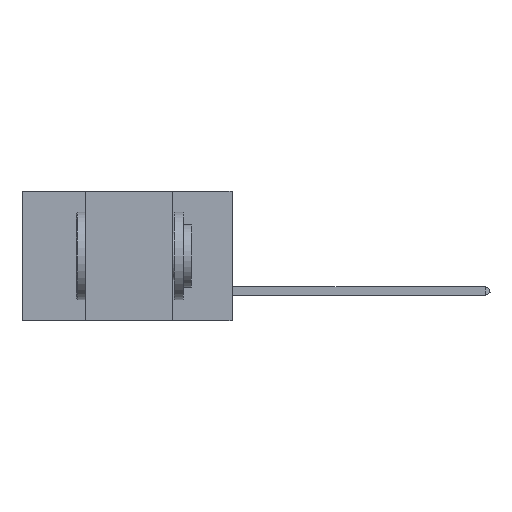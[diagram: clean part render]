
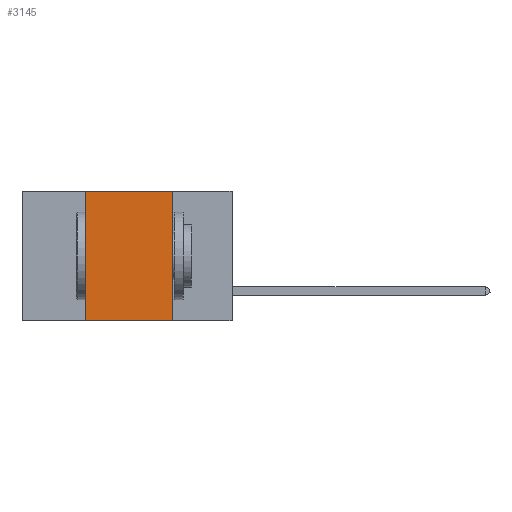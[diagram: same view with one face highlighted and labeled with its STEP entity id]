
A CAD part, left-side view. The second image highlights one B-rep face of the part: STEP entity #3145.
In plain terms, the highlighted planar face has unit normal (-1, 0, 0).
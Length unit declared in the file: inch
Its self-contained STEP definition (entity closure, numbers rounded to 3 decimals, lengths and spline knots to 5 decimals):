
#512 = DIRECTION ( 'NONE',  ( 0., -1., 0. ) ) ;
#902 = LINE ( 'NONE', #2764, #2570 ) ;
#1570 = FACE_OUTER_BOUND ( 'NONE', #9577, .T. ) ;
#2570 = VECTOR ( 'NONE', #2907, 39.37008 ) ;
#2736 = CARTESIAN_POINT ( 'NONE',  ( 0., 0.6, 0. ) ) ;
#2764 = CARTESIAN_POINT ( 'NONE',  ( 0., 0.42, 0. ) ) ;
#2907 = DIRECTION ( 'NONE',  ( 0., 0., 1. ) ) ;
#3134 = ORIENTED_EDGE ( 'NONE', *, *, #12017, .T. ) ;
#3145 = ADVANCED_FACE ( 'NONE', ( #1570 ), #3684, .F. ) ;
#3314 = LINE ( 'NONE', #2736, #4780 ) ;
#3684 = PLANE ( 'NONE',  #11522 ) ;
#4619 = ORIENTED_EDGE ( 'NONE', *, *, #10856, .F. ) ;
#4644 = CARTESIAN_POINT ( 'NONE',  ( 0., 0.17, -0.37 ) ) ;
#4731 = CARTESIAN_POINT ( 'NONE',  ( 0., 0.6, -0.37 ) ) ;
#4780 = VECTOR ( 'NONE', #10152, 39.37008 ) ;
#5534 = VERTEX_POINT ( 'NONE', #4644 ) ;
#5561 = EDGE_CURVE ( 'NONE', #11864, #7594, #3314, .T. ) ;
#6052 = LINE ( 'NONE', #4731, #12442 ) ;
#6476 = DIRECTION ( 'NONE',  ( 0., 0., -1. ) ) ;
#7594 = VERTEX_POINT ( 'NONE', #12583 ) ;
#8033 = EDGE_CURVE ( 'NONE', #8265, #11864, #902, .T. ) ;
#8153 = CARTESIAN_POINT ( 'NONE',  ( 0., 0.6, 0. ) ) ;
#8265 = VERTEX_POINT ( 'NONE', #8790 ) ;
#8790 = CARTESIAN_POINT ( 'NONE',  ( 0., 0.42, -0.37 ) ) ;
#8933 = ORIENTED_EDGE ( 'NONE', *, *, #8033, .F. ) ;
#9413 = LINE ( 'NONE', #12843, #11059 ) ;
#9577 = EDGE_LOOP ( 'NONE', ( #4619, #10728, #8933, #3134 ) ) ;
#10152 = DIRECTION ( 'NONE',  ( 0., -1., 0. ) ) ;
#10252 = DIRECTION ( 'NONE',  ( 0., 0., -1. ) ) ;
#10728 = ORIENTED_EDGE ( 'NONE', *, *, #5561, .F. ) ;
#10856 = EDGE_CURVE ( 'NONE', #7594, #5534, #9413, .T. ) ;
#11059 = VECTOR ( 'NONE', #6476, 39.37008 ) ;
#11445 = DIRECTION ( 'NONE',  ( 1., 0., 0. ) ) ;
#11522 = AXIS2_PLACEMENT_3D ( 'NONE', #8153, #11445, #10252 ) ;
#11597 = CARTESIAN_POINT ( 'NONE',  ( 0., 0.42, 0. ) ) ;
#11864 = VERTEX_POINT ( 'NONE', #11597 ) ;
#12017 = EDGE_CURVE ( 'NONE', #8265, #5534, #6052, .T. ) ;
#12442 = VECTOR ( 'NONE', #512, 39.37008 ) ;
#12583 = CARTESIAN_POINT ( 'NONE',  ( 0., 0.17, 0. ) ) ;
#12843 = CARTESIAN_POINT ( 'NONE',  ( 0., 0.17, 0. ) ) ;
